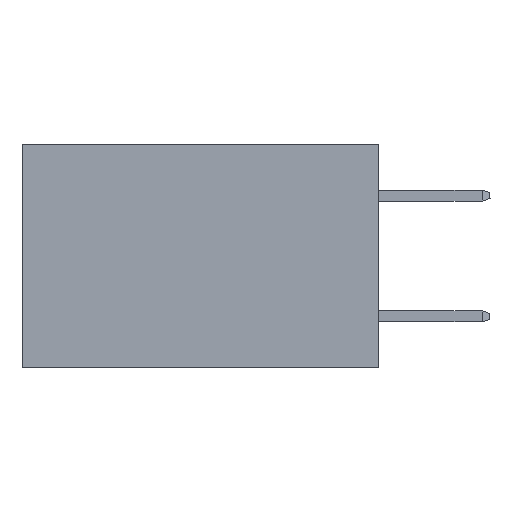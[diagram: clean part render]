
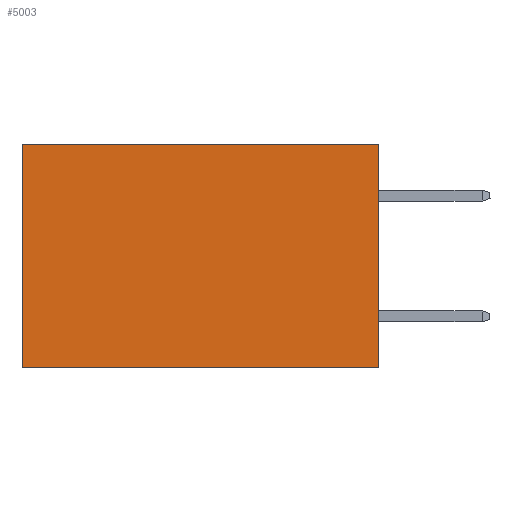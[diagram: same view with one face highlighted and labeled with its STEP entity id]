
A CAD part, left-side view. The second image highlights one B-rep face of the part: STEP entity #5003.
In plain terms, the highlighted planar face has unit normal (-1, 0, 0).
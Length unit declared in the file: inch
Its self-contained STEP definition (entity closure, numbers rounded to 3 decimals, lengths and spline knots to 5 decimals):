
#540 = VERTEX_POINT ( 'NONE', #15319 ) ;
#991 = CARTESIAN_POINT ( 'NONE',  ( 0.277, 0., 0. ) ) ;
#1169 = VERTEX_POINT ( 'NONE', #15157 ) ;
#1796 = DIRECTION ( 'NONE',  ( 0., 0., -1. ) ) ;
#1921 = VECTOR ( 'NONE', #9233, 39.37008 ) ;
#2751 = VECTOR ( 'NONE', #4067, 39.37008 ) ;
#2908 = CARTESIAN_POINT ( 'NONE',  ( 0.277, 0., -0.37 ) ) ;
#3260 = CARTESIAN_POINT ( 'NONE',  ( 0.277, 0.59, -0.37 ) ) ;
#4067 = DIRECTION ( 'NONE',  ( 0., 1., 0. ) ) ;
#4685 = AXIS2_PLACEMENT_3D ( 'NONE', #14834, #7374, #17871 ) ;
#5003 = ADVANCED_FACE ( 'NONE', ( #19288 ), #13297, .F. ) ;
#6113 = VECTOR ( 'NONE', #17688, 39.37008 ) ;
#6360 = EDGE_CURVE ( 'NONE', #540, #7827, #10558, .T. ) ;
#6988 = EDGE_CURVE ( 'NONE', #540, #1169, #14750, .T. ) ;
#7189 = CARTESIAN_POINT ( 'NONE',  ( 0.277, 0., -0.37 ) ) ;
#7374 = DIRECTION ( 'NONE',  ( 1., 0., 0. ) ) ;
#7729 = CARTESIAN_POINT ( 'NONE',  ( 0.277, 0., -0.37 ) ) ;
#7827 = VERTEX_POINT ( 'NONE', #2908 ) ;
#8743 = ORIENTED_EDGE ( 'NONE', *, *, #6988, .T. ) ;
#9060 = EDGE_LOOP ( 'NONE', ( #13571, #12018, #17892, #8743 ) ) ;
#9233 = DIRECTION ( 'NONE',  ( 0., 1., 0. ) ) ;
#9938 = VERTEX_POINT ( 'NONE', #3260 ) ;
#10558 = LINE ( 'NONE', #7189, #6113 ) ;
#10632 = EDGE_CURVE ( 'NONE', #7827, #9938, #13917, .T. ) ;
#10807 = CARTESIAN_POINT ( 'NONE',  ( 0.277, 0.59, -0.37 ) ) ;
#12018 = ORIENTED_EDGE ( 'NONE', *, *, #10632, .F. ) ;
#12825 = LINE ( 'NONE', #10807, #13769 ) ;
#12885 = EDGE_CURVE ( 'NONE', #1169, #9938, #12825, .T. ) ;
#13297 = PLANE ( 'NONE',  #4685 ) ;
#13571 = ORIENTED_EDGE ( 'NONE', *, *, #12885, .T. ) ;
#13769 = VECTOR ( 'NONE', #1796, 39.37008 ) ;
#13917 = LINE ( 'NONE', #7729, #1921 ) ;
#14750 = LINE ( 'NONE', #991, #2751 ) ;
#14834 = CARTESIAN_POINT ( 'NONE',  ( 0.277, 0., -0.37 ) ) ;
#15157 = CARTESIAN_POINT ( 'NONE',  ( 0.277, 0.59, 0. ) ) ;
#15319 = CARTESIAN_POINT ( 'NONE',  ( 0.277, 0., 0. ) ) ;
#17688 = DIRECTION ( 'NONE',  ( 0., 0., -1. ) ) ;
#17871 = DIRECTION ( 'NONE',  ( 0., 0., -1. ) ) ;
#17892 = ORIENTED_EDGE ( 'NONE', *, *, #6360, .F. ) ;
#19288 = FACE_OUTER_BOUND ( 'NONE', #9060, .T. ) ;
